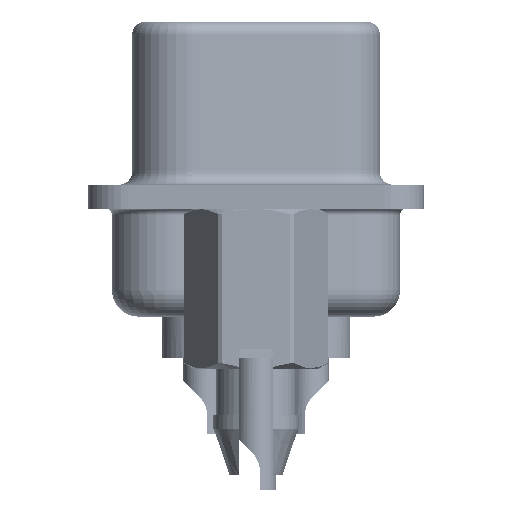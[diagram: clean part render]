
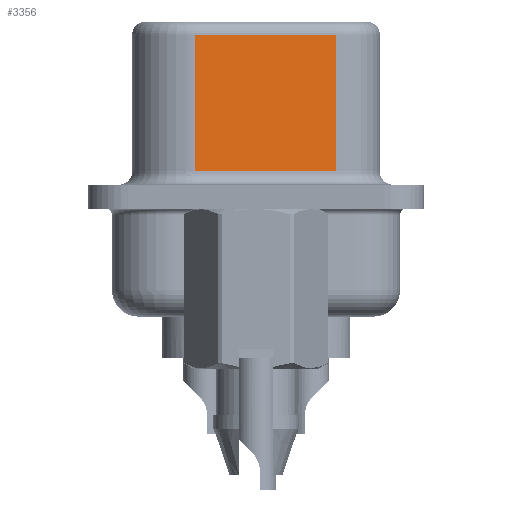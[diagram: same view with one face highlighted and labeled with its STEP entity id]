
A CAD part, left-side view. The second image highlights one B-rep face of the part: STEP entity #3356.
In plain terms, the highlighted planar face has unit normal (-0.985, -0.174, 0).
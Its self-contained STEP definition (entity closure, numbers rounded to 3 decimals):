
#86 = AXIS2_PLACEMENT_3D ( 'NONE', #19301, #36172, #5367 ) ;
#950 = CARTESIAN_POINT ( 'NONE',  ( 3.62, 2.293, 6.07 ) ) ;
#2230 = EDGE_CURVE ( 'NONE', #7477, #6701, #22093, .T. ) ;
#3356 = ADVANCED_FACE ( 'NONE', ( #19474 ), #30804, .F. ) ;
#5076 = VECTOR ( 'NONE', #20562, 1000. ) ;
#5201 = DIRECTION ( 'NONE',  ( 0., 0., -1. ) ) ;
#5310 = EDGE_CURVE ( 'NONE', #7477, #8632, #12015, .T. ) ;
#5367 = DIRECTION ( 'NONE',  ( -0.174, 0.985, 0. ) ) ;
#6701 = VERTEX_POINT ( 'NONE', #12290 ) ;
#6881 = ORIENTED_EDGE ( 'NONE', *, *, #16679, .T. ) ;
#7477 = VERTEX_POINT ( 'NONE', #9827 ) ;
#8632 = VERTEX_POINT ( 'NONE', #950 ) ;
#9827 = CARTESIAN_POINT ( 'NONE',  ( 4.551, -2.987, 6.07 ) ) ;
#12015 = LINE ( 'NONE', #34642, #5076 ) ;
#12290 = CARTESIAN_POINT ( 'NONE',  ( 4.551, -2.987, 0.95 ) ) ;
#13735 = EDGE_CURVE ( 'NONE', #25432, #6701, #25309, .T. ) ;
#16679 = EDGE_CURVE ( 'NONE', #8632, #25432, #33131, .T. ) ;
#16773 = CARTESIAN_POINT ( 'NONE',  ( 3.62, 2.293, 0.95 ) ) ;
#19301 = CARTESIAN_POINT ( 'NONE',  ( 4.551, -2.987, 6.57 ) ) ;
#19474 = FACE_OUTER_BOUND ( 'NONE', #33430, .T. ) ;
#20562 = DIRECTION ( 'NONE',  ( -0.174, 0.985, 0. ) ) ;
#21166 = ORIENTED_EDGE ( 'NONE', *, *, #5310, .T. ) ;
#21816 = DIRECTION ( 'NONE',  ( 0., 0., -1. ) ) ;
#21997 = CARTESIAN_POINT ( 'NONE',  ( 3.62, 2.293, 6.57 ) ) ;
#22093 = LINE ( 'NONE', #36559, #25740 ) ;
#25309 = LINE ( 'NONE', #30877, #27161 ) ;
#25432 = VERTEX_POINT ( 'NONE', #16773 ) ;
#25740 = VECTOR ( 'NONE', #5201, 1000. ) ;
#27161 = VECTOR ( 'NONE', #36618, 1000. ) ;
#29354 = ORIENTED_EDGE ( 'NONE', *, *, #2230, .F. ) ;
#30192 = VECTOR ( 'NONE', #21816, 1000. ) ;
#30697 = ORIENTED_EDGE ( 'NONE', *, *, #13735, .T. ) ;
#30804 = PLANE ( 'NONE',  #86 ) ;
#30877 = CARTESIAN_POINT ( 'NONE',  ( 4.551, -2.987, 0.95 ) ) ;
#33131 = LINE ( 'NONE', #21997, #30192 ) ;
#33430 = EDGE_LOOP ( 'NONE', ( #29354, #21166, #6881, #30697 ) ) ;
#34642 = CARTESIAN_POINT ( 'NONE',  ( 4.551, -2.987, 6.07 ) ) ;
#36172 = DIRECTION ( 'NONE',  ( 0.985, 0.174, 0. ) ) ;
#36559 = CARTESIAN_POINT ( 'NONE',  ( 4.551, -2.987, 6.57 ) ) ;
#36618 = DIRECTION ( 'NONE',  ( 0.174, -0.985, 0. ) ) ;
